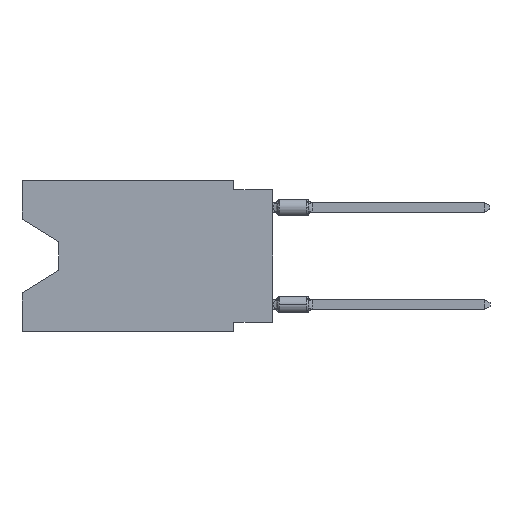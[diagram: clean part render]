
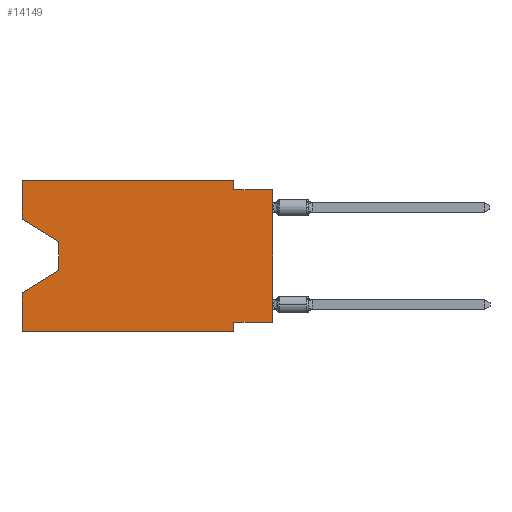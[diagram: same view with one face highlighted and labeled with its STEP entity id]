
A CAD part, left-side view. The second image highlights one B-rep face of the part: STEP entity #14149.
In plain terms, the highlighted planar face has unit normal (-1, 0, 0).
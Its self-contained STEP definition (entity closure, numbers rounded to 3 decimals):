
#262 = VECTOR ( 'NONE', #4451, 1000. ) ;
#462 = VERTEX_POINT ( 'NONE', #28356 ) ;
#464 = CARTESIAN_POINT ( 'NONE',  ( 0., 2.54, -9.271 ) ) ;
#815 = CARTESIAN_POINT ( 'NONE',  ( 0., 13.97, -5.893 ) ) ;
#930 = DIRECTION ( 'NONE',  ( 0., -1., 0. ) ) ;
#1638 = CARTESIAN_POINT ( 'NONE',  ( 0., 2.54, 0. ) ) ;
#1885 = CARTESIAN_POINT ( 'NONE',  ( 0., 13.97, -4.013 ) ) ;
#2499 = VERTEX_POINT ( 'NONE', #23546 ) ;
#2534 = DIRECTION ( 'NONE',  ( 0., 1., 0. ) ) ;
#2573 = VECTOR ( 'NONE', #9749, 1000. ) ;
#2587 = CARTESIAN_POINT ( 'NONE',  ( 0., 0., -0.635 ) ) ;
#3423 = VECTOR ( 'NONE', #13333, 1000. ) ;
#3720 = FACE_OUTER_BOUND ( 'NONE', #15905, .T. ) ;
#3854 = DIRECTION ( 'NONE',  ( 0., 0., -1. ) ) ;
#3915 = ORIENTED_EDGE ( 'NONE', *, *, #5097, .F. ) ;
#4406 = VECTOR ( 'NONE', #25217, 1000. ) ;
#4439 = VECTOR ( 'NONE', #24613, 1000. ) ;
#4451 = DIRECTION ( 'NONE',  ( 0., -1., 0. ) ) ;
#4822 = CARTESIAN_POINT ( 'NONE',  ( 0., 0., -9.271 ) ) ;
#4841 = VECTOR ( 'NONE', #16534, 1000. ) ;
#4899 = DIRECTION ( 'NONE',  ( 0., -1., 0. ) ) ;
#5088 = CARTESIAN_POINT ( 'NONE',  ( 0., 13.97, -5.893 ) ) ;
#5097 = EDGE_CURVE ( 'NONE', #9112, #462, #10405, .T. ) ;
#5786 = DIRECTION ( 'NONE',  ( 0., 0., -1. ) ) ;
#6310 = EDGE_CURVE ( 'NONE', #462, #26288, #26725, .T. ) ;
#6492 = EDGE_CURVE ( 'NONE', #20442, #18657, #18789, .T. ) ;
#6927 = EDGE_CURVE ( 'NONE', #17910, #18657, #11711, .T. ) ;
#7800 = LINE ( 'NONE', #16972, #19334 ) ;
#7922 = CARTESIAN_POINT ( 'NONE',  ( 0., 2.54, -9.906 ) ) ;
#8330 = CARTESIAN_POINT ( 'NONE',  ( 0., 16.383, -7.36 ) ) ;
#8566 = EDGE_CURVE ( 'NONE', #16098, #27995, #22472, .T. ) ;
#9112 = VERTEX_POINT ( 'NONE', #14639 ) ;
#9577 = VECTOR ( 'NONE', #930, 1000. ) ;
#9749 = DIRECTION ( 'NONE',  ( 0., 0., 1. ) ) ;
#9915 = VECTOR ( 'NONE', #19161, 1000. ) ;
#10405 = LINE ( 'NONE', #1638, #9915 ) ;
#10573 = EDGE_CURVE ( 'NONE', #27995, #17910, #7800, .T. ) ;
#10682 = ORIENTED_EDGE ( 'NONE', *, *, #6492, .F. ) ;
#11026 = ORIENTED_EDGE ( 'NONE', *, *, #6310, .F. ) ;
#11404 = CARTESIAN_POINT ( 'NONE',  ( 0., 16.383, 0. ) ) ;
#11549 = CARTESIAN_POINT ( 'NONE',  ( 0., 16.383, -2.546 ) ) ;
#11711 = LINE ( 'NONE', #815, #4406 ) ;
#12353 = LINE ( 'NONE', #7922, #4841 ) ;
#12946 = ORIENTED_EDGE ( 'NONE', *, *, #26070, .T. ) ;
#13333 = DIRECTION ( 'NONE',  ( 0., 0., 1. ) ) ;
#13406 = ORIENTED_EDGE ( 'NONE', *, *, #18724, .T. ) ;
#13620 = LINE ( 'NONE', #13894, #3423 ) ;
#13894 = CARTESIAN_POINT ( 'NONE',  ( 0., 0., 0. ) ) ;
#14149 = ADVANCED_FACE ( 'NONE', ( #3720 ), #25693, .F. ) ;
#14639 = CARTESIAN_POINT ( 'NONE',  ( 0., 2.54, 0. ) ) ;
#15496 = ORIENTED_EDGE ( 'NONE', *, *, #16702, .F. ) ;
#15724 = EDGE_CURVE ( 'NONE', #2499, #26369, #22048, .T. ) ;
#15905 = EDGE_LOOP ( 'NONE', ( #23033, #18623, #23889, #10682, #12946, #21083, #20633, #13406, #11026, #3915, #15496, #19035 ) ) ;
#16098 = VERTEX_POINT ( 'NONE', #27670 ) ;
#16352 = CARTESIAN_POINT ( 'NONE',  ( 0., 16.383, 0. ) ) ;
#16534 = DIRECTION ( 'NONE',  ( 0., 0., -1. ) ) ;
#16702 = EDGE_CURVE ( 'NONE', #19789, #9112, #24566, .T. ) ;
#16972 = CARTESIAN_POINT ( 'NONE',  ( 0., 13.97, -4.013 ) ) ;
#17061 = VERTEX_POINT ( 'NONE', #20044 ) ;
#17386 = AXIS2_PLACEMENT_3D ( 'NONE', #23515, #21222, #3854 ) ;
#17887 = EDGE_CURVE ( 'NONE', #16098, #19789, #22877, .T. ) ;
#17910 = VERTEX_POINT ( 'NONE', #5088 ) ;
#18623 = ORIENTED_EDGE ( 'NONE', *, *, #10573, .T. ) ;
#18657 = VERTEX_POINT ( 'NONE', #8330 ) ;
#18724 = EDGE_CURVE ( 'NONE', #2499, #26288, #13620, .T. ) ;
#18789 = LINE ( 'NONE', #16352, #2573 ) ;
#19035 = ORIENTED_EDGE ( 'NONE', *, *, #17887, .F. ) ;
#19161 = DIRECTION ( 'NONE',  ( 0., 0., -1. ) ) ;
#19334 = VECTOR ( 'NONE', #5786, 1000. ) ;
#19576 = EDGE_CURVE ( 'NONE', #26369, #17061, #12353, .T. ) ;
#19789 = VERTEX_POINT ( 'NONE', #21965 ) ;
#20044 = CARTESIAN_POINT ( 'NONE',  ( 0., 2.54, -9.906 ) ) ;
#20307 = DIRECTION ( 'NONE',  ( 0., -0.855, -0.519 ) ) ;
#20442 = VERTEX_POINT ( 'NONE', #23055 ) ;
#20584 = LINE ( 'NONE', #27357, #9577 ) ;
#20633 = ORIENTED_EDGE ( 'NONE', *, *, #15724, .F. ) ;
#21083 = ORIENTED_EDGE ( 'NONE', *, *, #19576, .F. ) ;
#21222 = DIRECTION ( 'NONE',  ( 1., 0., 0. ) ) ;
#21699 = CARTESIAN_POINT ( 'NONE',  ( 0., 0., -0.635 ) ) ;
#21965 = CARTESIAN_POINT ( 'NONE',  ( 0., 16.383, 0. ) ) ;
#22048 = LINE ( 'NONE', #4822, #26169 ) ;
#22415 = CARTESIAN_POINT ( 'NONE',  ( 0., 16.383, 0. ) ) ;
#22472 = LINE ( 'NONE', #11549, #26140 ) ;
#22877 = LINE ( 'NONE', #11404, #4439 ) ;
#23033 = ORIENTED_EDGE ( 'NONE', *, *, #8566, .T. ) ;
#23055 = CARTESIAN_POINT ( 'NONE',  ( 0., 16.383, -9.906 ) ) ;
#23515 = CARTESIAN_POINT ( 'NONE',  ( 0., 16.383, 0. ) ) ;
#23546 = CARTESIAN_POINT ( 'NONE',  ( 0., 0., -9.271 ) ) ;
#23889 = ORIENTED_EDGE ( 'NONE', *, *, #6927, .T. ) ;
#24566 = LINE ( 'NONE', #22415, #28051 ) ;
#24613 = DIRECTION ( 'NONE',  ( 0., 0., 1. ) ) ;
#25217 = DIRECTION ( 'NONE',  ( 0., 0.855, -0.519 ) ) ;
#25693 = PLANE ( 'NONE',  #17386 ) ;
#26070 = EDGE_CURVE ( 'NONE', #20442, #17061, #20584, .T. ) ;
#26140 = VECTOR ( 'NONE', #20307, 1000. ) ;
#26169 = VECTOR ( 'NONE', #2534, 1000. ) ;
#26288 = VERTEX_POINT ( 'NONE', #21699 ) ;
#26369 = VERTEX_POINT ( 'NONE', #464 ) ;
#26725 = LINE ( 'NONE', #2587, #262 ) ;
#27357 = CARTESIAN_POINT ( 'NONE',  ( 0., 16.383, -9.906 ) ) ;
#27670 = CARTESIAN_POINT ( 'NONE',  ( 0., 16.383, -2.546 ) ) ;
#27995 = VERTEX_POINT ( 'NONE', #1885 ) ;
#28051 = VECTOR ( 'NONE', #4899, 1000. ) ;
#28356 = CARTESIAN_POINT ( 'NONE',  ( 0., 2.54, -0.635 ) ) ;
